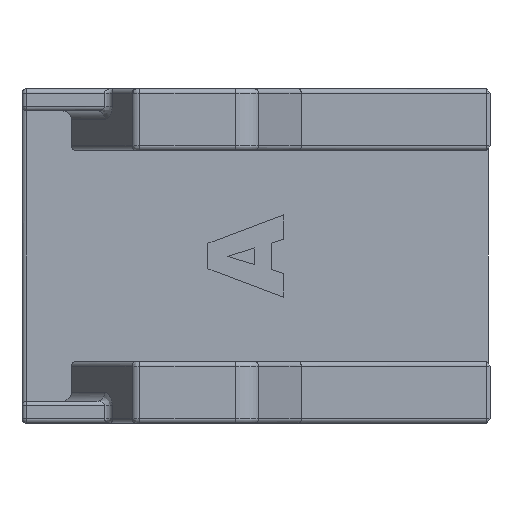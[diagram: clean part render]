
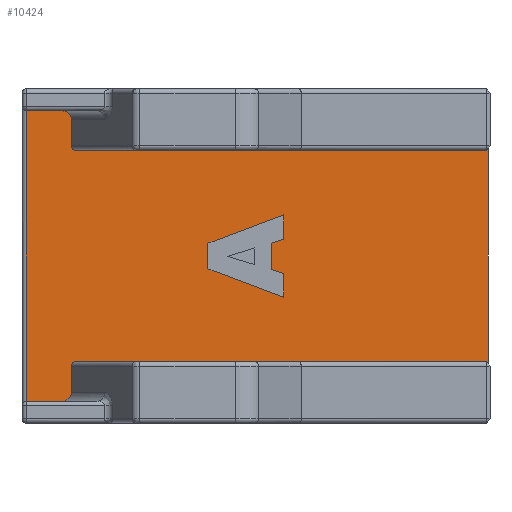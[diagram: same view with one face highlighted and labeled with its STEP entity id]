
A CAD part, left-side view. The second image highlights one B-rep face of the part: STEP entity #10424.
In plain terms, the highlighted planar face has unit normal (-1, 0, 0).
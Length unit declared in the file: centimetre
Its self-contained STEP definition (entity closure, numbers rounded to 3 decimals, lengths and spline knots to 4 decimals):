
#1095=ELLIPSE($,#11096,0.0577,0.05);
#1096=ELLIPSE($,#11097,0.1155,0.1);
#1097=ELLIPSE($,#11098,0.1155,0.1);
#1098=ELLIPSE($,#11099,0.0577,0.05);
#1259=FACE_BOUND($,#1962,.T.);
#1297=FACE_OUTER_BOUND($,#1961,.T.);
#1961=EDGE_LOOP($,(#6997,#6998,#6999,#7000,#7001,#7002,#7003,#7004,#7005,
#7006,#7007,#7008,#7009,#7010));
#1962=EDGE_LOOP($,(#7011,#7012,#7013,#7014,#7015,#7016,#7017,#7018));
#2642=LINE($,#14881,#3491);
#2646=LINE($,#14889,#3495);
#2649=LINE($,#14895,#3498);
#2652=LINE($,#14901,#3501);
#2664=LINE($,#14924,#3513);
#2666=LINE($,#14928,#3515);
#2668=LINE($,#14932,#3517);
#2670=LINE($,#14935,#3519);
#2671=LINE($,#14939,#3520);
#2672=LINE($,#14941,#3521);
#2673=LINE($,#14943,#3522);
#2674=LINE($,#14947,#3523);
#2675=LINE($,#14951,#3524);
#2676=LINE($,#14953,#3525);
#2677=LINE($,#14955,#3526);
#2678=LINE($,#14959,#3527);
#2679=LINE($,#14963,#3528);
#2680=LINE($,#14964,#3529);
#3491=VECTOR($,#12071,0.9177);
#3495=VECTOR($,#12077,0.2895);
#3498=VECTOR($,#12082,0.9176);
#3501=VECTOR($,#12087,0.278);
#3513=VECTOR($,#12107,0.1482);
#3515=VECTOR($,#12111,0.3013);
#3517=VECTOR($,#12115,0.1478);
#3519=VECTOR($,#12119,0.271);
#3520=VECTOR($,#12122,2.48);
#3521=VECTOR($,#12123,0.0567);
#3522=VECTOR($,#12124,4.6385);
#3523=VECTOR($,#12127,0.3);
#3524=VECTOR($,#12130,0.3963);
#3525=VECTOR($,#12131,3.3);
#3526=VECTOR($,#12132,0.3963);
#3527=VECTOR($,#12135,0.3);
#3528=VECTOR($,#12138,4.6385);
#3529=VECTOR($,#12139,0.0567);
#4340=VERTEX_POINT($,#14879);
#4341=VERTEX_POINT($,#14880);
#4344=VERTEX_POINT($,#14888);
#4346=VERTEX_POINT($,#14894);
#4348=VERTEX_POINT($,#14900);
#4355=VERTEX_POINT($,#14923);
#4356=VERTEX_POINT($,#14927);
#4357=VERTEX_POINT($,#14931);
#4358=VERTEX_POINT($,#14937);
#4359=VERTEX_POINT($,#14938);
#4360=VERTEX_POINT($,#14940);
#4361=VERTEX_POINT($,#14942);
#4362=VERTEX_POINT($,#14944);
#4363=VERTEX_POINT($,#14946);
#4364=VERTEX_POINT($,#14948);
#4365=VERTEX_POINT($,#14950);
#4366=VERTEX_POINT($,#14952);
#4367=VERTEX_POINT($,#14954);
#4368=VERTEX_POINT($,#14956);
#4369=VERTEX_POINT($,#14958);
#4370=VERTEX_POINT($,#14960);
#4371=VERTEX_POINT($,#14962);
#5314=EDGE_CURVE($,#4340,#4341,#2642,.T.);
#5318=EDGE_CURVE($,#4341,#4344,#2646,.T.);
#5321=EDGE_CURVE($,#4344,#4346,#2649,.T.);
#5324=EDGE_CURVE($,#4346,#4348,#2652,.T.);
#5336=EDGE_CURVE($,#4348,#4355,#2664,.T.);
#5338=EDGE_CURVE($,#4355,#4356,#2666,.T.);
#5340=EDGE_CURVE($,#4356,#4357,#2668,.T.);
#5342=EDGE_CURVE($,#4357,#4340,#2670,.T.);
#5343=EDGE_CURVE($,#4358,#4359,#2671,.F.);
#5344=EDGE_CURVE($,#4360,#4359,#2672,.F.);
#5345=EDGE_CURVE($,#4361,#4360,#2673,.T.);
#5346=EDGE_CURVE($,#4362,#4361,#1095,.F.);
#5347=EDGE_CURVE($,#4362,#4363,#2674,.T.);
#5348=EDGE_CURVE($,#4363,#4364,#1096,.T.);
#5349=EDGE_CURVE($,#4365,#4364,#2675,.T.);
#5350=EDGE_CURVE($,#4366,#4365,#2676,.T.);
#5351=EDGE_CURVE($,#4367,#4366,#2677,.T.);
#5352=EDGE_CURVE($,#4367,#4368,#1097,.T.);
#5353=EDGE_CURVE($,#4368,#4369,#2678,.T.);
#5354=EDGE_CURVE($,#4370,#4369,#1098,.F.);
#5355=EDGE_CURVE($,#4371,#4370,#2679,.T.);
#5356=EDGE_CURVE($,#4358,#4371,#2680,.F.);
#6997=ORIENTED_EDGE($,*,*,#5343,.T.);
#6998=ORIENTED_EDGE($,*,*,#5344,.F.);
#6999=ORIENTED_EDGE($,*,*,#5345,.F.);
#7000=ORIENTED_EDGE($,*,*,#5346,.F.);
#7001=ORIENTED_EDGE($,*,*,#5347,.T.);
#7002=ORIENTED_EDGE($,*,*,#5348,.T.);
#7003=ORIENTED_EDGE($,*,*,#5349,.F.);
#7004=ORIENTED_EDGE($,*,*,#5350,.F.);
#7005=ORIENTED_EDGE($,*,*,#5351,.F.);
#7006=ORIENTED_EDGE($,*,*,#5352,.T.);
#7007=ORIENTED_EDGE($,*,*,#5353,.T.);
#7008=ORIENTED_EDGE($,*,*,#5354,.F.);
#7009=ORIENTED_EDGE($,*,*,#5355,.F.);
#7010=ORIENTED_EDGE($,*,*,#5356,.F.);
#7011=ORIENTED_EDGE($,*,*,#5336,.T.);
#7012=ORIENTED_EDGE($,*,*,#5338,.T.);
#7013=ORIENTED_EDGE($,*,*,#5340,.T.);
#7014=ORIENTED_EDGE($,*,*,#5342,.T.);
#7015=ORIENTED_EDGE($,*,*,#5314,.T.);
#7016=ORIENTED_EDGE($,*,*,#5318,.T.);
#7017=ORIENTED_EDGE($,*,*,#5321,.T.);
#7018=ORIENTED_EDGE($,*,*,#5324,.T.);
#10218=PLANE($,#11095);
#10424=ADVANCED_FACE($,(#1297,#1259),#10218,.F.);
#11095=AXIS2_PLACEMENT_3D($,#14936,#12120,#12121);
#11096=AXIS2_PLACEMENT_3D($,#14945,#12125,#12126);
#11097=AXIS2_PLACEMENT_3D($,#14949,#12128,#12129);
#11098=AXIS2_PLACEMENT_3D($,#14957,#12133,#12134);
#11099=AXIS2_PLACEMENT_3D($,#14961,#12136,#12137);
#12071=DIRECTION($,(0.,0.936,0.352));
#12077=DIRECTION($,(0.,0.,1.));
#12082=DIRECTION($,(0.,-0.936,0.352));
#12087=DIRECTION($,(0.,0.,-1.));
#12107=DIRECTION($,(0.,0.957,-0.29));
#12111=DIRECTION($,(0.,0.,-1.));
#12115=DIRECTION($,(0.,-0.959,-0.283));
#12119=DIRECTION($,(0.,0.,-1.));
#12120=DIRECTION('center_axis',(1.,0.,0.));
#12121=DIRECTION('ref_axis',(0.,0.,-1.));
#12122=DIRECTION($,(0.,0.,-1.));
#12123=DIRECTION($,(0.,0.708,-0.706));
#12124=DIRECTION($,(0.,-1.,0.));
#12125=DIRECTION('center_axis',(1.,0.,0.));
#12126=DIRECTION('ref_axis',(0.,1.,0.));
#12127=DIRECTION($,(0.,0.,1.));
#12128=DIRECTION('center_axis',(-1.,0.,0.));
#12129=DIRECTION('ref_axis',(0.,-1.,0.));
#12130=DIRECTION($,(0.,-1.,0.));
#12131=DIRECTION($,(0.,0.,1.));
#12132=DIRECTION($,(0.,1.,0.));
#12133=DIRECTION('center_axis',(-1.,0.,0.));
#12134=DIRECTION('ref_axis',(0.,-1.,0.));
#12135=DIRECTION($,(0.,0.,1.));
#12136=DIRECTION('center_axis',(1.,0.,0.));
#12137=DIRECTION('ref_axis',(0.,1.,0.));
#12138=DIRECTION($,(0.,1.,0.));
#12139=DIRECTION($,(0.,-0.708,-0.706));
#14879=CARTESIAN_POINT('',(-8.24,-3.8006,-0.3682));
#14880=CARTESIAN_POINT('',(-8.24,-2.9416,-0.0453));
#14881=CARTESIAN_POINT($,(-8.24,-2.9932,-0.0647));
#14888=CARTESIAN_POINT('',(-8.24,-2.9416,0.2442));
#14889=CARTESIAN_POINT($,(-8.24,-2.9416,0.1721));
#14894=CARTESIAN_POINT('',(-8.24,-3.8006,0.567));
#14895=CARTESIAN_POINT($,(-8.24,-3.4229,0.4251));
#14900=CARTESIAN_POINT('',(-8.24,-3.8006,0.289));
#14901=CARTESIAN_POINT($,(-8.24,-3.8006,0.1945));
#14923=CARTESIAN_POINT('',(-8.24,-3.6588,0.246));
#14924=CARTESIAN_POINT($,(-8.24,-3.3891,0.1643));
#14927=CARTESIAN_POINT('',(-8.24,-3.6588,-0.0553));
#14928=CARTESIAN_POINT($,(-8.24,-3.6588,0.0223));
#14931=CARTESIAN_POINT('',(-8.24,-3.8006,-0.0972));
#14932=CARTESIAN_POINT($,(-8.24,-3.4581,0.0039));
#14935=CARTESIAN_POINT($,(-8.24,-3.8006,-0.1341));
#14936=CARTESIAN_POINT('Origin',(-8.24,-3.1141,0.1));
#14937=CARTESIAN_POINT('',(-8.24,-6.1271,-1.14));
#14938=CARTESIAN_POINT('',(-8.24,-6.1271,1.34));
#14939=CARTESIAN_POINT($,(-8.24,-6.1271,0.1));
#14940=CARTESIAN_POINT('',(-8.24,-6.0869,1.3));
#14941=CARTESIAN_POINT($,(-8.24,-4.9611,0.1784));
#14942=CARTESIAN_POINT('',(-8.24,-1.4485,1.3));
#14943=CARTESIAN_POINT($,(-8.24,-3.284,1.3));
#14944=CARTESIAN_POINT('',(-8.24,-1.3907,1.35));
#14945=CARTESIAN_POINT('Origin',(-8.24,-1.4485,1.35));
#14946=CARTESIAN_POINT('',(-8.24,-1.3907,1.65));
#14947=CARTESIAN_POINT($,(-8.24,-1.3907,-0.91));
#14948=CARTESIAN_POINT('',(-8.24,-1.2753,1.75));
#14949=CARTESIAN_POINT('Origin',(-8.24,-1.2753,1.65));
#14950=CARTESIAN_POINT('',(-8.24,-0.879,1.75));
#14951=CARTESIAN_POINT($,(-8.24,-3.284,1.75));
#14952=CARTESIAN_POINT('',(-8.24,-0.879,-1.55));
#14953=CARTESIAN_POINT($,(-8.24,-0.879,0.1));
#14954=CARTESIAN_POINT('',(-8.24,-1.2753,-1.55));
#14955=CARTESIAN_POINT($,(-8.24,-3.1547,-1.55));
#14956=CARTESIAN_POINT('',(-8.24,-1.3907,-1.45));
#14957=CARTESIAN_POINT('Origin',(-8.24,-1.2753,-1.45));
#14958=CARTESIAN_POINT('',(-8.24,-1.3907,-1.15));
#14959=CARTESIAN_POINT($,(-8.24,-1.3907,-0.91));
#14960=CARTESIAN_POINT('',(-8.24,-1.4485,-1.1));
#14961=CARTESIAN_POINT('Origin',(-8.24,-1.4485,-1.15));
#14962=CARTESIAN_POINT('',(-8.24,-6.0869,-1.1));
#14963=CARTESIAN_POINT($,(-8.24,-3.1547,-1.1));
#14964=CARTESIAN_POINT($,(-8.24,-5.0099,-0.027));
